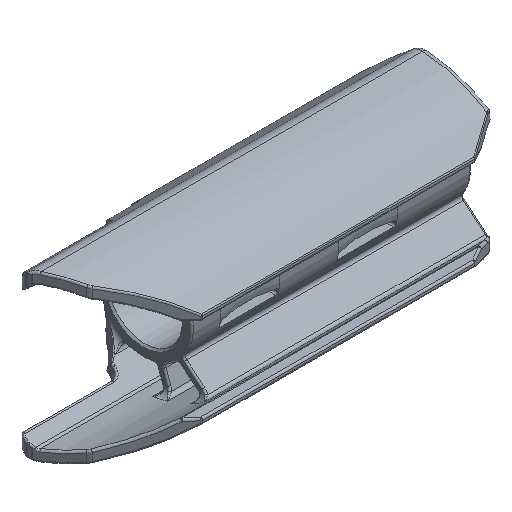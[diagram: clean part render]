
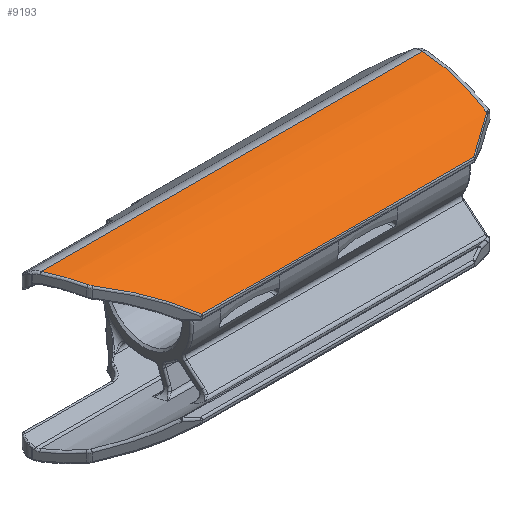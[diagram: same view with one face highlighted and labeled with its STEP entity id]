
A CAD part, isometric view. The second image highlights one B-rep face of the part: STEP entity #9193.
In plain terms, the highlighted cylindrical face has radius 57.15 mm (diameter 114.3 mm), a partial arc.
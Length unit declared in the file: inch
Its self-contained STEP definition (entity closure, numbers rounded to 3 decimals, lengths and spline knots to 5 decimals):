
#23 = CARTESIAN_POINT ( 'NONE',  ( 7., 0.03063, -0.84991 ) ) ;
#179 = CARTESIAN_POINT ( 'NONE',  ( 7., -0.09092, 1.39681 ) ) ;
#191 = EDGE_CURVE ( 'NONE', #13406, #2953, #11874, .T. ) ;
#870 = LINE ( 'NONE', #9100, #9849 ) ;
#953 = CARTESIAN_POINT ( 'NONE',  ( 1.75727, -1.48987, 0.80858 ) ) ;
#971 = EDGE_LOOP ( 'NONE', ( #6426, #3526, #1072, #3914, #2128, #3840, #12612 ) ) ;
#1072 = ORIENTED_EDGE ( 'NONE', *, *, #2124, .F. ) ;
#1124 = CARTESIAN_POINT ( 'NONE',  ( 0.72168, -0.59619, 1.31102 ) ) ;
#1327 = DIRECTION ( 'NONE',  ( 0., -0.296, 0.955 ) ) ;
#1790 = LINE ( 'NONE', #179, #5621 ) ;
#2011 = CARTESIAN_POINT ( 'NONE',  ( 6.9, -1.17837, 1.04768 ) ) ;
#2020 = EDGE_CURVE ( 'NONE', #2953, #9991, #4606, .T. ) ;
#2122 = CARTESIAN_POINT ( 'NONE',  ( 1.12695, -0.95352, 1.20019 ) ) ;
#2124 = EDGE_CURVE ( 'NONE', #7474, #9523, #11334, .T. ) ;
#2128 = ORIENTED_EDGE ( 'NONE', *, *, #5222, .F. ) ;
#2233 = B_SPLINE_CURVE_WITH_KNOTS ( 'NONE', 3,
 ( #2250, #4611, #8120, #1124 ),
 .UNSPECIFIED., .F., .F.,
 ( 4, 4 ),
 ( 0., 1. ),
 .UNSPECIFIED. ) ;
#2250 = CARTESIAN_POINT ( 'NONE',  ( 0.75656, -0.63835, 1.29834 ) ) ;
#2375 = DIRECTION ( 'NONE',  ( 1., 0., 0. ) ) ;
#2889 = AXIS2_PLACEMENT_3D ( 'NONE', #5707, #10062, #1327 ) ;
#2953 = VERTEX_POINT ( 'NONE', #2011 ) ;
#3289 = CARTESIAN_POINT ( 'NONE',  ( 6.9, -1.17837, 1.04768 ) ) ;
#3526 = ORIENTED_EDGE ( 'NONE', *, *, #14718, .F. ) ;
#3840 = ORIENTED_EDGE ( 'NONE', *, *, #6117, .F. ) ;
#3861 = VERTEX_POINT ( 'NONE', #9455 ) ;
#3914 = ORIENTED_EDGE ( 'NONE', *, *, #12481, .F. ) ;
#4236 = CARTESIAN_POINT ( 'NONE',  ( 0.43401, -0.09092, 1.39681 ) ) ;
#4479 = CARTESIAN_POINT ( 'NONE',  ( 0.53134, -0.26187, 1.38756 ) ) ;
#4606 = B_SPLINE_CURVE_WITH_KNOTS ( 'NONE', 3,
 ( #3289, #10006, #5679, #9621 ),
 .UNSPECIFIED., .F., .F.,
 ( 4, 4 ),
 ( 0., 1. ),
 .UNSPECIFIED. ) ;
#4611 = CARTESIAN_POINT ( 'NONE',  ( 0.74255, -0.62643, 1.30205 ) ) ;
#4725 = DIRECTION ( 'NONE',  ( 0., -0.68, 0.733 ) ) ;
#5222 = EDGE_CURVE ( 'NONE', #3861, #7133, #6550, .T. ) ;
#5225 = CYLINDRICAL_SURFACE ( 'NONE', #10698, 2.25 ) ;
#5621 = VECTOR ( 'NONE', #8198, 39.37008 ) ;
#5679 = CARTESIAN_POINT ( 'NONE',  ( 6.53276, -1.39326, 0.89715 ) ) ;
#5707 = CARTESIAN_POINT ( 'NONE',  ( 6.9, 0.03063, -0.84991 ) ) ;
#6117 = EDGE_CURVE ( 'NONE', #9991, #3861, #870, .T. ) ;
#6364 = CARTESIAN_POINT ( 'NONE',  ( 6.9, -0.09092, 1.39681 ) ) ;
#6426 = ORIENTED_EDGE ( 'NONE', *, *, #191, .F. ) ;
#6550 = B_SPLINE_CURVE_WITH_KNOTS ( 'NONE', 3,
 ( #953, #7939, #2122, #10311 ),
 .UNSPECIFIED., .F., .F.,
 ( 4, 4 ),
 ( 0., 1. ),
 .UNSPECIFIED. ) ;
#7133 = VERTEX_POINT ( 'NONE', #7682 ) ;
#7474 = VERTEX_POINT ( 'NONE', #10873 ) ;
#7682 = CARTESIAN_POINT ( 'NONE',  ( 0.75656, -0.63835, 1.29834 ) ) ;
#7797 = DIRECTION ( 'NONE',  ( -1., 0., 0. ) ) ;
#7939 = CARTESIAN_POINT ( 'NONE',  ( 1.47132, -1.24655, 1.03165 ) ) ;
#8120 = CARTESIAN_POINT ( 'NONE',  ( 0.73073, -0.61208, 1.30641 ) ) ;
#8198 = DIRECTION ( 'NONE',  ( 1., 0., 0. ) ) ;
#9100 = CARTESIAN_POINT ( 'NONE',  ( 7., -1.48987, 0.80858 ) ) ;
#9193 = ADVANCED_FACE ( 'NONE', ( #14600 ), #5225, .T. ) ;
#9455 = CARTESIAN_POINT ( 'NONE',  ( 1.75727, -1.48987, 0.80858 ) ) ;
#9479 = CARTESIAN_POINT ( 'NONE',  ( 0.72168, -0.59619, 1.31102 ) ) ;
#9523 = VERTEX_POINT ( 'NONE', #4236 ) ;
#9621 = CARTESIAN_POINT ( 'NONE',  ( 6.36766, -1.48987, 0.80858 ) ) ;
#9849 = VECTOR ( 'NONE', #7797, 39.37008 ) ;
#9991 = VERTEX_POINT ( 'NONE', #11073 ) ;
#10006 = CARTESIAN_POINT ( 'NONE',  ( 6.71111, -1.2889, 0.97725 ) ) ;
#10062 = DIRECTION ( 'NONE',  ( 1., 0., 0. ) ) ;
#10311 = CARTESIAN_POINT ( 'NONE',  ( 0.75656, -0.63835, 1.29834 ) ) ;
#10698 = AXIS2_PLACEMENT_3D ( 'NONE', #23, #2375, #4725 ) ;
#10873 = CARTESIAN_POINT ( 'NONE',  ( 0.72168, -0.59619, 1.31102 ) ) ;
#11073 = CARTESIAN_POINT ( 'NONE',  ( 6.36766, -1.48987, 0.80858 ) ) ;
#11334 = B_SPLINE_CURVE_WITH_KNOTS ( 'NONE', 3,
 ( #9479, #11475, #4479, #12751 ),
 .UNSPECIFIED., .F., .F.,
 ( 4, 4 ),
 ( 0., 1. ),
 .UNSPECIFIED. ) ;
#11475 = CARTESIAN_POINT ( 'NONE',  ( 0.62807, -0.43176, 1.35871 ) ) ;
#11874 = CIRCLE ( 'NONE', #2889, 2.25 ) ;
#12481 = EDGE_CURVE ( 'NONE', #7133, #7474, #2233, .T. ) ;
#12612 = ORIENTED_EDGE ( 'NONE', *, *, #2020, .F. ) ;
#12751 = CARTESIAN_POINT ( 'NONE',  ( 0.43401, -0.09092, 1.39681 ) ) ;
#13406 = VERTEX_POINT ( 'NONE', #6364 ) ;
#14600 = FACE_OUTER_BOUND ( 'NONE', #971, .T. ) ;
#14718 = EDGE_CURVE ( 'NONE', #9523, #13406, #1790, .T. ) ;
